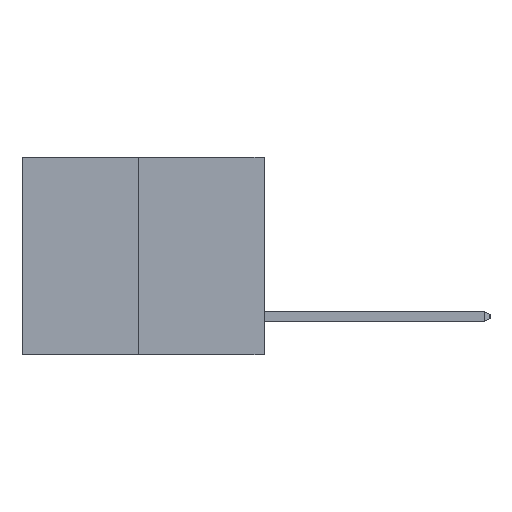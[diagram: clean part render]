
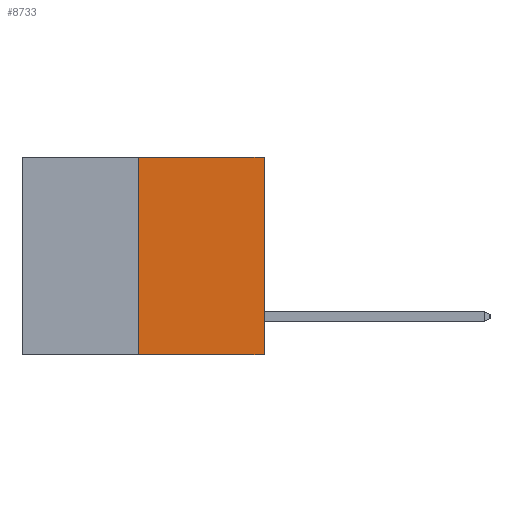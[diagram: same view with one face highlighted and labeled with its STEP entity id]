
A CAD part, left-side view. The second image highlights one B-rep face of the part: STEP entity #8733.
In plain terms, the highlighted planar face has unit normal (-1, 0, 0).
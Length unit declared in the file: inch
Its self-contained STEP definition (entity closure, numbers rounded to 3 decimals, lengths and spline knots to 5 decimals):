
#172 = VERTEX_POINT ( 'NONE', #14793 ) ;
#618 = EDGE_CURVE ( 'NONE', #172, #8812, #16734, .T. ) ;
#1234 = LINE ( 'NONE', #14698, #17557 ) ;
#2104 = AXIS2_PLACEMENT_3D ( 'NONE', #19153, #19212, #16102 ) ;
#3466 = LINE ( 'NONE', #9421, #4685 ) ;
#4179 = VERTEX_POINT ( 'NONE', #17424 ) ;
#4685 = VECTOR ( 'NONE', #7875, 39.37008 ) ;
#4722 = ORIENTED_EDGE ( 'NONE', *, *, #5822, .T. ) ;
#4977 = LINE ( 'NONE', #5630, #13707 ) ;
#5630 = CARTESIAN_POINT ( 'NONE',  ( 0., 0.312, -0.49 ) ) ;
#5822 = EDGE_CURVE ( 'NONE', #8812, #15050, #1234, .T. ) ;
#6090 = ORIENTED_EDGE ( 'NONE', *, *, #618, .T. ) ;
#6241 = ORIENTED_EDGE ( 'NONE', *, *, #12742, .F. ) ;
#6475 = FACE_OUTER_BOUND ( 'NONE', #18354, .T. ) ;
#7389 = DIRECTION ( 'NONE',  ( 0., -1., 0. ) ) ;
#7875 = DIRECTION ( 'NONE',  ( 0., -1., 0. ) ) ;
#8733 = ADVANCED_FACE ( 'NONE', ( #6475 ), #14531, .F. ) ;
#8809 = CARTESIAN_POINT ( 'NONE',  ( 0., 0., -0.49 ) ) ;
#8812 = VERTEX_POINT ( 'NONE', #8809 ) ;
#8939 = VECTOR ( 'NONE', #7389, 39.37008 ) ;
#9421 = CARTESIAN_POINT ( 'NONE',  ( 0., 0.6, 0. ) ) ;
#10428 = CARTESIAN_POINT ( 'NONE',  ( 0., 0.6, -0.49 ) ) ;
#12742 = EDGE_CURVE ( 'NONE', #4179, #15050, #3466, .T. ) ;
#13707 = VECTOR ( 'NONE', #17965, 39.37008 ) ;
#14012 = ORIENTED_EDGE ( 'NONE', *, *, #16778, .F. ) ;
#14531 = PLANE ( 'NONE',  #2104 ) ;
#14698 = CARTESIAN_POINT ( 'NONE',  ( 0., 0., 0. ) ) ;
#14793 = CARTESIAN_POINT ( 'NONE',  ( 0., 0.312, -0.49 ) ) ;
#15050 = VERTEX_POINT ( 'NONE', #19343 ) ;
#16102 = DIRECTION ( 'NONE',  ( 0., 0., -1. ) ) ;
#16734 = LINE ( 'NONE', #10428, #8939 ) ;
#16778 = EDGE_CURVE ( 'NONE', #172, #4179, #4977, .T. ) ;
#17424 = CARTESIAN_POINT ( 'NONE',  ( 0., 0.312, 0. ) ) ;
#17557 = VECTOR ( 'NONE', #17829, 39.37008 ) ;
#17829 = DIRECTION ( 'NONE',  ( 0., 0., 1. ) ) ;
#17965 = DIRECTION ( 'NONE',  ( 0., 0., 1. ) ) ;
#18354 = EDGE_LOOP ( 'NONE', ( #14012, #6090, #4722, #6241 ) ) ;
#19153 = CARTESIAN_POINT ( 'NONE',  ( 0., 0.6, 0. ) ) ;
#19212 = DIRECTION ( 'NONE',  ( 1., 0., 0. ) ) ;
#19343 = CARTESIAN_POINT ( 'NONE',  ( 0., 0., 0. ) ) ;
